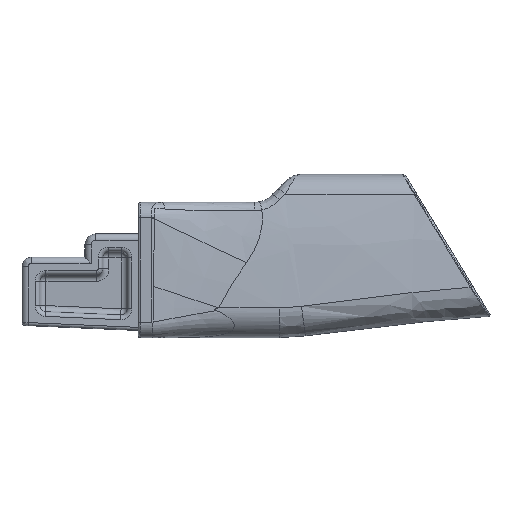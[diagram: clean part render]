
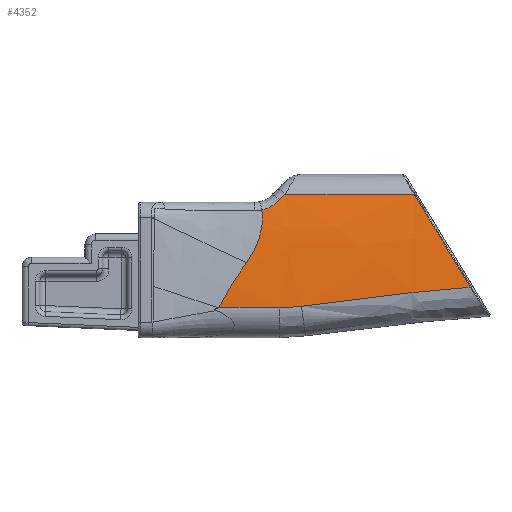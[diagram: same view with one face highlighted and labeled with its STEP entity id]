
A CAD part, left-side view. The second image highlights one B-rep face of the part: STEP entity #4352.
In plain terms, the highlighted free-form (B-spline) face has degree [1, 2] with [2, 3] control points.
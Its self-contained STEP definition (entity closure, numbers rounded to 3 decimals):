
#94=(
BOUNDED_SURFACE()
B_SPLINE_SURFACE(1,2,((#10169,#10170,#10171),(#10172,#10173,#10174)),
 .UNSPECIFIED.,.F.,.F.,.F.)
B_SPLINE_SURFACE_WITH_KNOTS((2,2),(3,3),(1.952,3.152),
(-2.476,-1.817),.UNSPECIFIED.)
GEOMETRIC_REPRESENTATION_ITEM()
RATIONAL_B_SPLINE_SURFACE(((1.,0.946,1.),(1.,0.946,
1.)))
REPRESENTATION_ITEM('')
SURFACE()
);
#338=LINE('',#9989,#529);
#343=LINE('',#10175,#534);
#529=VECTOR('',#6031,10.);
#534=VECTOR('',#6062,10.);
#920=FACE_OUTER_BOUND('',#1219,.T.);
#1219=EDGE_LOOP('',(#3962,#3963,#3964,#3965,#3966,#3967,#3968,#3969,#3970,
#3971,#3972,#3973,#3974,#3975));
#1237=B_SPLINE_CURVE_WITH_KNOTS('',3,(#6350,#6351,#6352,#6353),
 .UNSPECIFIED.,.F.,.F.,(4,4),(0.,0.034),.UNSPECIFIED.);
#1239=B_SPLINE_CURVE_WITH_KNOTS('',3,(#6382,#6383,#6384,#6385,#6386),
 .UNSPECIFIED.,.F.,.F.,(4,1,4),(0.,1.496,3.49),
 .UNSPECIFIED.);
#1241=B_SPLINE_CURVE_WITH_KNOTS('',3,(#6407,#6408,#6409,#6410),
 .UNSPECIFIED.,.F.,.F.,(4,4),(0.,0.009),
 .UNSPECIFIED.);
#1281=B_SPLINE_CURVE_WITH_KNOTS('',3,(#7033,#7034,#7035,#7036),
 .UNSPECIFIED.,.F.,.F.,(4,4),(-5.463,-5.368),
 .UNSPECIFIED.);
#1282=B_SPLINE_CURVE_WITH_KNOTS('',3,(#7038,#7039,#7040,#7041),
 .UNSPECIFIED.,.F.,.F.,(4,4),(-5.368,-3.576),
 .UNSPECIFIED.);
#1283=B_SPLINE_CURVE_WITH_KNOTS('',3,(#7043,#7044,#7045,#7046),
 .UNSPECIFIED.,.F.,.F.,(4,4),(-3.576,0.),.UNSPECIFIED.);
#1357=B_SPLINE_CURVE_WITH_KNOTS('',3,(#9436,#9437,#9438,#9439,#9440,#9441,
#9442),.UNSPECIFIED.,.F.,.F.,(4,1,1,1,4),(0.,0.977,1.955,
2.932,3.125),.UNSPECIFIED.);
#1358=B_SPLINE_CURVE_WITH_KNOTS('',3,(#9465,#9466,#9467,#9468,#9469),
 .UNSPECIFIED.,.F.,.F.,(4,1,4),(23.985,24.996,26.344),
 .UNSPECIFIED.);
#1368=B_SPLINE_CURVE_WITH_KNOTS('',3,(#10049,#10050,#10051,#10052),
 .UNSPECIFIED.,.F.,.F.,(4,4),(-0.712,0.),.UNSPECIFIED.);
#1370=B_SPLINE_CURVE_WITH_KNOTS('',3,(#10130,#10131,#10132,#10133),
 .UNSPECIFIED.,.F.,.F.,(4,4),(-0.253,0.),.UNSPECIFIED.);
#1371=B_SPLINE_CURVE_WITH_KNOTS('',3,(#10155,#10156,#10157,#10158),
 .UNSPECIFIED.,.F.,.F.,(4,4),(-0.412,0.),.UNSPECIFIED.);
#1372=B_SPLINE_CURVE_WITH_KNOTS('',3,(#10159,#10160,#10161,#10162),
 .UNSPECIFIED.,.F.,.F.,(4,4),(-0.662,-0.412),
 .UNSPECIFIED.);
#1674=VERTEX_POINT('',#6285);
#1676=VERTEX_POINT('',#6340);
#1679=VERTEX_POINT('',#6348);
#1680=VERTEX_POINT('',#6374);
#1722=VERTEX_POINT('',#7032);
#1723=VERTEX_POINT('',#7037);
#1724=VERTEX_POINT('',#7042);
#1934=VERTEX_POINT('',#9224);
#1940=VERTEX_POINT('',#9434);
#1941=VERTEX_POINT('',#9463);
#2024=VERTEX_POINT('',#9987);
#2031=VERTEX_POINT('',#10105);
#2032=VERTEX_POINT('',#10128);
#2033=VERTEX_POINT('',#10154);
#2064=EDGE_CURVE('',#1679,#1676,#1237,.T.);
#2067=EDGE_CURVE('',#1676,#1680,#1239,.T.);
#2069=EDGE_CURVE('',#1674,#1679,#1241,.T.);
#2135=EDGE_CURVE('',#1680,#1722,#1281,.T.);
#2136=EDGE_CURVE('',#1722,#1723,#1282,.T.);
#2137=EDGE_CURVE('',#1723,#1724,#1283,.T.);
#2494=EDGE_CURVE('',#1940,#1934,#1357,.T.);
#2496=EDGE_CURVE('',#1941,#1940,#1358,.T.);
#2662=EDGE_CURVE('',#2024,#1941,#338,.T.);
#2672=EDGE_CURVE('',#1724,#2024,#1368,.T.);
#2678=EDGE_CURVE('',#2032,#2031,#1370,.T.);
#2679=EDGE_CURVE('',#2033,#2032,#1371,.T.);
#2680=EDGE_CURVE('',#1934,#2033,#1372,.T.);
#2683=EDGE_CURVE('',#1674,#2031,#343,.T.);
#3962=ORIENTED_EDGE('',*,*,#2069,.F.);
#3963=ORIENTED_EDGE('',*,*,#2683,.T.);
#3964=ORIENTED_EDGE('',*,*,#2678,.F.);
#3965=ORIENTED_EDGE('',*,*,#2679,.F.);
#3966=ORIENTED_EDGE('',*,*,#2680,.F.);
#3967=ORIENTED_EDGE('',*,*,#2494,.F.);
#3968=ORIENTED_EDGE('',*,*,#2496,.F.);
#3969=ORIENTED_EDGE('',*,*,#2662,.F.);
#3970=ORIENTED_EDGE('',*,*,#2672,.F.);
#3971=ORIENTED_EDGE('',*,*,#2137,.F.);
#3972=ORIENTED_EDGE('',*,*,#2136,.F.);
#3973=ORIENTED_EDGE('',*,*,#2135,.F.);
#3974=ORIENTED_EDGE('',*,*,#2067,.F.);
#3975=ORIENTED_EDGE('',*,*,#2064,.F.);
#4352=ADVANCED_FACE('',(#920),#94,.T.);
#6031=DIRECTION('',(0.,1.,0.));
#6062=DIRECTION('',(0.,1.,0.));
#6285=CARTESIAN_POINT('',(-10.031,-547.989,133.253));
#6340=CARTESIAN_POINT('',(-10.141,-548.208,132.893));
#6348=CARTESIAN_POINT('',(-10.054,-548.035,133.179));
#6350=CARTESIAN_POINT('Ctrl Pts',(-10.054,-548.035,133.179));
#6351=CARTESIAN_POINT('Ctrl Pts',(-10.083,-548.092,133.084));
#6352=CARTESIAN_POINT('Ctrl Pts',(-10.112,-548.15,132.988));
#6353=CARTESIAN_POINT('Ctrl Pts',(-10.141,-548.208,132.893));
#6374=CARTESIAN_POINT('',(-15.267,-566.13,103.355));
#6382=CARTESIAN_POINT('Ctrl Pts',(-10.141,-548.208,132.893));
#6383=CARTESIAN_POINT('Ctrl Pts',(-11.394,-550.718,128.749));
#6384=CARTESIAN_POINT('Ctrl Pts',(-13.545,-556.669,118.939));
#6385=CARTESIAN_POINT('Ctrl Pts',(-14.768,-562.685,109.029));
#6386=CARTESIAN_POINT('Ctrl Pts',(-15.267,-566.13,103.355));
#6407=CARTESIAN_POINT('Ctrl Pts',(-10.031,-547.989,133.253));
#6408=CARTESIAN_POINT('Ctrl Pts',(-10.038,-548.004,133.229));
#6409=CARTESIAN_POINT('Ctrl Pts',(-10.046,-548.02,133.204));
#6410=CARTESIAN_POINT('Ctrl Pts',(-10.054,-548.035,133.179));
#7032=CARTESIAN_POINT('',(-15.274,-565.183,103.279));
#7033=CARTESIAN_POINT('Ctrl Pts',(-15.267,-566.13,103.355));
#7034=CARTESIAN_POINT('Ctrl Pts',(-15.269,-565.814,103.33));
#7035=CARTESIAN_POINT('Ctrl Pts',(-15.272,-565.499,103.304));
#7036=CARTESIAN_POINT('Ctrl Pts',(-15.274,-565.183,103.279));
#7037=CARTESIAN_POINT('',(-15.412,-547.336,101.634));
#7038=CARTESIAN_POINT('Ctrl Pts',(-15.274,-565.183,103.279));
#7039=CARTESIAN_POINT('Ctrl Pts',(-15.317,-559.229,102.793));
#7040=CARTESIAN_POINT('Ctrl Pts',(-15.363,-553.28,102.245));
#7041=CARTESIAN_POINT('Ctrl Pts',(-15.413,-547.336,101.634));
#7042=CARTESIAN_POINT('',(-15.728,-511.831,97.222));
#7043=CARTESIAN_POINT('Ctrl Pts',(-15.413,-547.336,101.634));
#7044=CARTESIAN_POINT('Ctrl Pts',(-15.511,-535.474,100.413));
#7045=CARTESIAN_POINT('Ctrl Pts',(-15.62,-523.636,98.942));
#7046=CARTESIAN_POINT('Ctrl Pts',(-15.728,-511.831,97.222));
#9224=CARTESIAN_POINT('',(-11.416,-499.135,128.202));
#9434=CARTESIAN_POINT('',(-14.433,-494.201,111.229));
#9436=CARTESIAN_POINT('Ctrl Pts',(-14.433,-494.201,111.229));
#9437=CARTESIAN_POINT('Ctrl Pts',(-14.201,-495.567,113.086));
#9438=CARTESIAN_POINT('Ctrl Pts',(-13.67,-497.725,116.903));
#9439=CARTESIAN_POINT('Ctrl Pts',(-12.713,-499.322,122.403));
#9440=CARTESIAN_POINT('Ctrl Pts',(-11.929,-499.431,126.074));
#9441=CARTESIAN_POINT('Ctrl Pts',(-11.489,-499.185,127.905));
#9442=CARTESIAN_POINT('Ctrl Pts',(-11.416,-499.136,128.202));
#9463=CARTESIAN_POINT('',(-15.76,-485.341,96.708));
#9465=CARTESIAN_POINT('Ctrl Pts',(-15.76,-485.341,96.708));
#9466=CARTESIAN_POINT('Ctrl Pts',(-15.626,-486.392,98.922));
#9467=CARTESIAN_POINT('Ctrl Pts',(-15.251,-489.155,103.977));
#9468=CARTESIAN_POINT('Ctrl Pts',(-14.754,-492.311,108.661));
#9469=CARTESIAN_POINT('Ctrl Pts',(-14.433,-494.201,111.229));
#9987=CARTESIAN_POINT('',(-15.76,-504.734,96.708));
#9989=CARTESIAN_POINT('',(-15.76,-697.501,96.708));
#10049=CARTESIAN_POINT('Ctrl Pts',(-15.728,-511.831,
97.222));
#10050=CARTESIAN_POINT('Ctrl Pts',(-15.75,-509.481,
96.88));
#10051=CARTESIAN_POINT('Ctrl Pts',(-15.76,-507.108,
96.708));
#10052=CARTESIAN_POINT('Ctrl Pts',(-15.76,-504.734,
96.708));
#10105=CARTESIAN_POINT('',(-10.031,-506.567,133.253));
#10128=CARTESIAN_POINT('',(-10.569,-504.818,131.424));
#10130=CARTESIAN_POINT('Ctrl Pts',(-10.569,-504.818,
131.424));
#10131=CARTESIAN_POINT('Ctrl Pts',(-10.398,-505.402,132.033));
#10132=CARTESIAN_POINT('Ctrl Pts',(-10.219,-505.985,
132.643));
#10133=CARTESIAN_POINT('Ctrl Pts',(-10.031,-506.567,133.253));
#10154=CARTESIAN_POINT('',(-11.212,-501.496,129.02));
#10155=CARTESIAN_POINT('Ctrl Pts',(-11.212,-501.494,
129.023));
#10156=CARTESIAN_POINT('Ctrl Pts',(-11.062,-502.733,
129.616));
#10157=CARTESIAN_POINT('Ctrl Pts',(-10.849,-503.866,
130.432));
#10158=CARTESIAN_POINT('Ctrl Pts',(-10.569,-504.818,
131.424));
#10159=CARTESIAN_POINT('Ctrl Pts',(-11.416,-499.135,128.202));
#10160=CARTESIAN_POINT('Ctrl Pts',(-11.371,-499.949,
128.385));
#10161=CARTESIAN_POINT('Ctrl Pts',(-11.303,-500.741,
128.663));
#10162=CARTESIAN_POINT('Ctrl Pts',(-11.212,-501.494,
129.023));
#10169=CARTESIAN_POINT('Ctrl Pts',(-10.031,-566.13,
133.253));
#10170=CARTESIAN_POINT('Ctrl Pts',(-14.405,-566.13,
119.04));
#10171=CARTESIAN_POINT('Ctrl Pts',(-15.76,-566.13,
96.708));
#10172=CARTESIAN_POINT('Ctrl Pts',(-10.031,-485.341,
133.253));
#10173=CARTESIAN_POINT('Ctrl Pts',(-14.405,-485.341,
119.04));
#10174=CARTESIAN_POINT('Ctrl Pts',(-15.76,-485.341,
96.708));
#10175=CARTESIAN_POINT('',(-10.031,-697.501,133.253));
